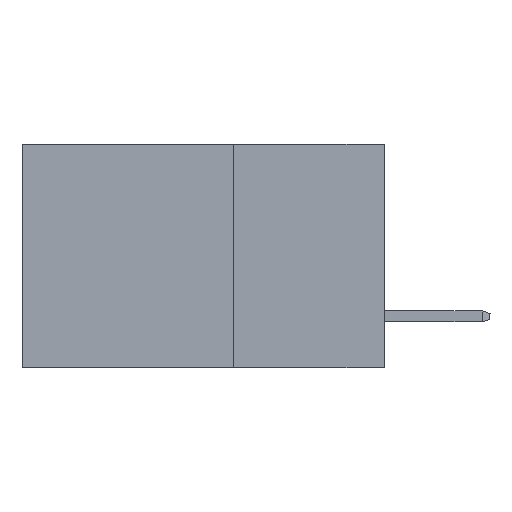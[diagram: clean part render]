
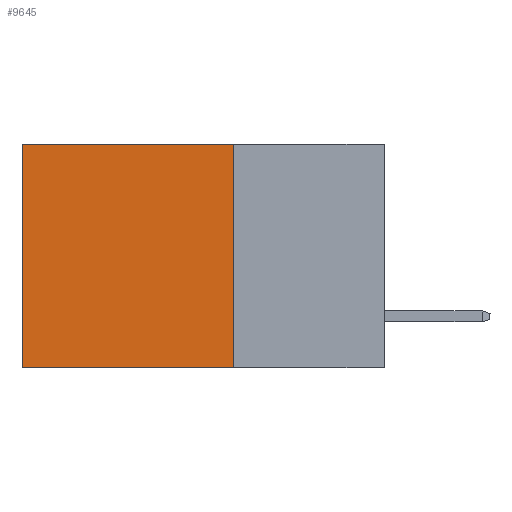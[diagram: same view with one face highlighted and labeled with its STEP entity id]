
A CAD part, left-side view. The second image highlights one B-rep face of the part: STEP entity #9645.
In plain terms, the highlighted planar face has unit normal (-1, 0, 0).
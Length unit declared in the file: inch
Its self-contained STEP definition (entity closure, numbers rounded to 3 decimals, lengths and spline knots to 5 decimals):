
#348 = DIRECTION ( 'NONE',  ( 0., 0., -1. ) ) ;
#466 = DIRECTION ( 'NONE',  ( 0., 1., 0. ) ) ;
#717 = VERTEX_POINT ( 'NONE', #9842 ) ;
#837 = PLANE ( 'NONE',  #7985 ) ;
#1138 = CARTESIAN_POINT ( 'NONE',  ( 0.2615, 0.6, -0.37 ) ) ;
#2884 = ORIENTED_EDGE ( 'NONE', *, *, #3424, .F. ) ;
#3424 = EDGE_CURVE ( 'NONE', #7359, #717, #7797, .T. ) ;
#3479 = EDGE_LOOP ( 'NONE', ( #4912, #2884, #3723, #7459 ) ) ;
#3573 = VECTOR ( 'NONE', #466, 39.37008 ) ;
#3723 = ORIENTED_EDGE ( 'NONE', *, *, #8227, .F. ) ;
#3950 = VERTEX_POINT ( 'NONE', #6480 ) ;
#4105 = DIRECTION ( 'NONE',  ( 0., 0., -1. ) ) ;
#4446 = LINE ( 'NONE', #7461, #3573 ) ;
#4549 = EDGE_CURVE ( 'NONE', #3950, #6240, #4446, .T. ) ;
#4691 = CARTESIAN_POINT ( 'NONE',  ( 0.2615, 0.25, -0.37 ) ) ;
#4718 = FACE_OUTER_BOUND ( 'NONE', #3479, .T. ) ;
#4798 = CARTESIAN_POINT ( 'NONE',  ( 0.2615, 0.25, -0.37 ) ) ;
#4895 = DIRECTION ( 'NONE',  ( 0., 1., 0. ) ) ;
#4912 = ORIENTED_EDGE ( 'NONE', *, *, #6452, .T. ) ;
#5765 = VECTOR ( 'NONE', #348, 39.37008 ) ;
#6240 = VERTEX_POINT ( 'NONE', #7642 ) ;
#6275 = CARTESIAN_POINT ( 'NONE',  ( 0.2615, 0.25, -0.37 ) ) ;
#6278 = DIRECTION ( 'NONE',  ( 0., 0., -1. ) ) ;
#6452 = EDGE_CURVE ( 'NONE', #6240, #717, #8680, .T. ) ;
#6480 = CARTESIAN_POINT ( 'NONE',  ( 0.2615, 0.25, 0. ) ) ;
#7080 = LINE ( 'NONE', #9481, #8324 ) ;
#7359 = VERTEX_POINT ( 'NONE', #4798 ) ;
#7459 = ORIENTED_EDGE ( 'NONE', *, *, #4549, .T. ) ;
#7461 = CARTESIAN_POINT ( 'NONE',  ( 0.2615, 0.25, 0. ) ) ;
#7642 = CARTESIAN_POINT ( 'NONE',  ( 0.2615, 0.6, 0. ) ) ;
#7797 = LINE ( 'NONE', #4691, #9758 ) ;
#7985 = AXIS2_PLACEMENT_3D ( 'NONE', #6275, #8602, #4105 ) ;
#8227 = EDGE_CURVE ( 'NONE', #3950, #7359, #7080, .T. ) ;
#8324 = VECTOR ( 'NONE', #6278, 39.37008 ) ;
#8602 = DIRECTION ( 'NONE',  ( 1., 0., 0. ) ) ;
#8680 = LINE ( 'NONE', #1138, #5765 ) ;
#9481 = CARTESIAN_POINT ( 'NONE',  ( 0.2615, 0.25, -0.37 ) ) ;
#9645 = ADVANCED_FACE ( 'NONE', ( #4718 ), #837, .F. ) ;
#9758 = VECTOR ( 'NONE', #4895, 39.37008 ) ;
#9842 = CARTESIAN_POINT ( 'NONE',  ( 0.2615, 0.6, -0.37 ) ) ;
